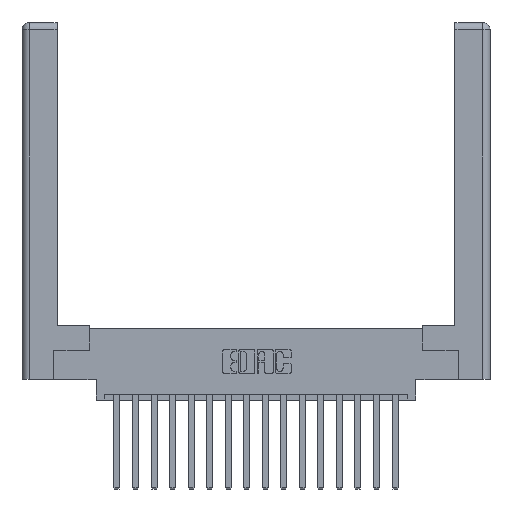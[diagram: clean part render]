
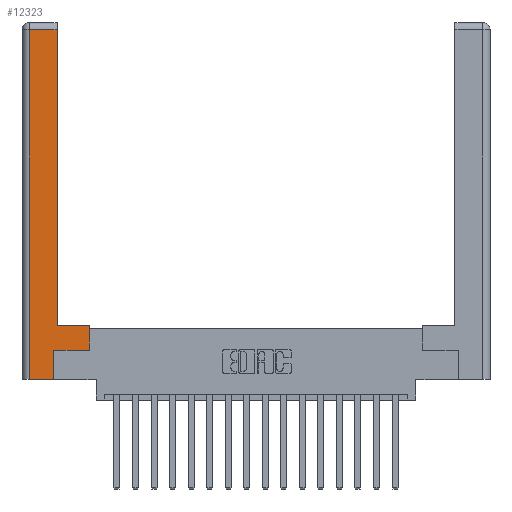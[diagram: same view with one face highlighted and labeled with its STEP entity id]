
A CAD part, top view. The second image highlights one B-rep face of the part: STEP entity #12323.
In plain terms, the highlighted planar face has unit normal (0, 0, 1).
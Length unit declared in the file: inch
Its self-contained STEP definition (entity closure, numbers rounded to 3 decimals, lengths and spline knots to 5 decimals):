
#76 = EDGE_CURVE ( 'NONE', #2157, #3755, #11581, .T. ) ;
#180 = LINE ( 'NONE', #11400, #10774 ) ;
#786 = CARTESIAN_POINT ( 'NONE',  ( 0.295, 2.94, 0. ) ) ;
#810 = VECTOR ( 'NONE', #7143, 39.37008 ) ;
#926 = VERTEX_POINT ( 'NONE', #17761 ) ;
#1032 = LINE ( 'NONE', #3593, #14528 ) ;
#1113 = EDGE_CURVE ( 'NONE', #8930, #5062, #15067, .T. ) ;
#1158 = VERTEX_POINT ( 'NONE', #9612 ) ;
#1363 = VECTOR ( 'NONE', #1824, 39.37008 ) ;
#1656 = ORIENTED_EDGE ( 'NONE', *, *, #1113, .T. ) ;
#1708 = LINE ( 'NONE', #14233, #14961 ) ;
#1824 = DIRECTION ( 'NONE',  ( -1., 0., 0. ) ) ;
#1957 = CARTESIAN_POINT ( 'NONE',  ( 0.295, 0.45, 0. ) ) ;
#2157 = VERTEX_POINT ( 'NONE', #9741 ) ;
#2165 = ORIENTED_EDGE ( 'NONE', *, *, #9391, .T. ) ;
#2532 = CARTESIAN_POINT ( 'NONE',  ( 0.265, 0., 0. ) ) ;
#3022 = EDGE_CURVE ( 'NONE', #7029, #2157, #12539, .T. ) ;
#3593 = CARTESIAN_POINT ( 'NONE',  ( 0.0615, 0., 0. ) ) ;
#3755 = VERTEX_POINT ( 'NONE', #7241 ) ;
#3820 = ORIENTED_EDGE ( 'NONE', *, *, #15520, .T. ) ;
#4054 = CARTESIAN_POINT ( 'NONE',  ( 0.265, 0.245, 0. ) ) ;
#5062 = VERTEX_POINT ( 'NONE', #8552 ) ;
#5249 = EDGE_CURVE ( 'NONE', #1158, #7029, #1032, .T. ) ;
#5823 = EDGE_CURVE ( 'NONE', #5062, #16204, #14759, .T. ) ;
#6485 = ORIENTED_EDGE ( 'NONE', *, *, #5823, .T. ) ;
#6919 = DIRECTION ( 'NONE',  ( -1., 0., 0. ) ) ;
#7029 = VERTEX_POINT ( 'NONE', #15749 ) ;
#7143 = DIRECTION ( 'NONE',  ( 0., 1., 0. ) ) ;
#7145 = DIRECTION ( 'NONE',  ( 0., 1., 0. ) ) ;
#7241 = CARTESIAN_POINT ( 'NONE',  ( 0.265, 0.245, 0. ) ) ;
#7433 = CARTESIAN_POINT ( 'NONE',  ( 0., 0., 0. ) ) ;
#8552 = CARTESIAN_POINT ( 'NONE',  ( 0.295, 0.45, 0. ) ) ;
#8632 = CARTESIAN_POINT ( 'NONE',  ( 0.565, 0.45, 0. ) ) ;
#8930 = VERTEX_POINT ( 'NONE', #8632 ) ;
#9307 = DIRECTION ( 'NONE',  ( 0., -1., 0. ) ) ;
#9391 = EDGE_CURVE ( 'NONE', #16204, #1158, #14125, .T. ) ;
#9612 = CARTESIAN_POINT ( 'NONE',  ( 0.0615, 2.94, 0. ) ) ;
#9741 = CARTESIAN_POINT ( 'NONE',  ( 0.265, 0., 0. ) ) ;
#9803 = EDGE_LOOP ( 'NONE', ( #6485, #2165, #12908, #11776, #14747, #17111, #3820, #1656 ) ) ;
#9845 = DIRECTION ( 'NONE',  ( 1., 0., 0. ) ) ;
#9962 = FACE_OUTER_BOUND ( 'NONE', #9803, .T. ) ;
#10280 = DIRECTION ( 'NONE',  ( -1., 0., 0. ) ) ;
#10774 = VECTOR ( 'NONE', #7145, 39.37008 ) ;
#11184 = EDGE_CURVE ( 'NONE', #3755, #926, #1708, .T. ) ;
#11400 = CARTESIAN_POINT ( 'NONE',  ( 0.565, 0.45, 0. ) ) ;
#11581 = LINE ( 'NONE', #4054, #12213 ) ;
#11776 = ORIENTED_EDGE ( 'NONE', *, *, #3022, .T. ) ;
#12213 = VECTOR ( 'NONE', #18175, 39.37008 ) ;
#12323 = ADVANCED_FACE ( 'NONE', ( #9962 ), #17186, .F. ) ;
#12326 = DIRECTION ( 'NONE',  ( 1., 0., 0. ) ) ;
#12539 = LINE ( 'NONE', #2532, #16551 ) ;
#12908 = ORIENTED_EDGE ( 'NONE', *, *, #5249, .T. ) ;
#13464 = VECTOR ( 'NONE', #6919, 39.37008 ) ;
#14125 = LINE ( 'NONE', #15261, #13464 ) ;
#14233 = CARTESIAN_POINT ( 'NONE',  ( 0.565, 0.245, 0. ) ) ;
#14528 = VECTOR ( 'NONE', #9307, 39.37008 ) ;
#14747 = ORIENTED_EDGE ( 'NONE', *, *, #76, .T. ) ;
#14759 = LINE ( 'NONE', #15752, #810 ) ;
#14961 = VECTOR ( 'NONE', #9845, 39.37008 ) ;
#15067 = LINE ( 'NONE', #1957, #1363 ) ;
#15261 = CARTESIAN_POINT ( 'NONE',  ( 0.0615, 2.94, 0. ) ) ;
#15520 = EDGE_CURVE ( 'NONE', #926, #8930, #180, .T. ) ;
#15749 = CARTESIAN_POINT ( 'NONE',  ( 0.0615, 0., 0. ) ) ;
#15752 = CARTESIAN_POINT ( 'NONE',  ( 0.295, 3., 0. ) ) ;
#16204 = VERTEX_POINT ( 'NONE', #786 ) ;
#16551 = VECTOR ( 'NONE', #12326, 39.37008 ) ;
#17111 = ORIENTED_EDGE ( 'NONE', *, *, #11184, .T. ) ;
#17186 = PLANE ( 'NONE',  #18050 ) ;
#17372 = DIRECTION ( 'NONE',  ( 0., 0., -1. ) ) ;
#17761 = CARTESIAN_POINT ( 'NONE',  ( 0.565, 0.245, 0. ) ) ;
#18050 = AXIS2_PLACEMENT_3D ( 'NONE', #7433, #17372, #10280 ) ;
#18175 = DIRECTION ( 'NONE',  ( 0., 1., 0. ) ) ;
